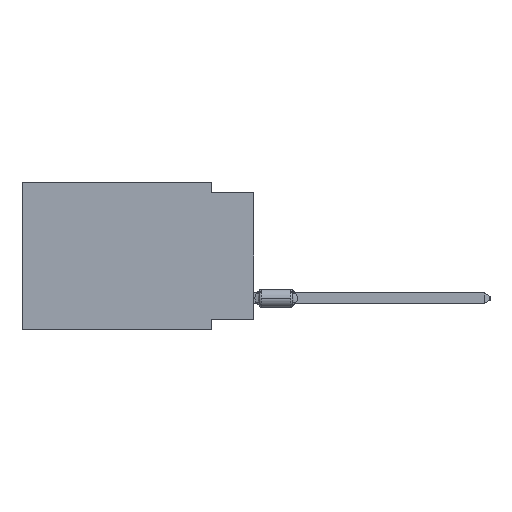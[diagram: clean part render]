
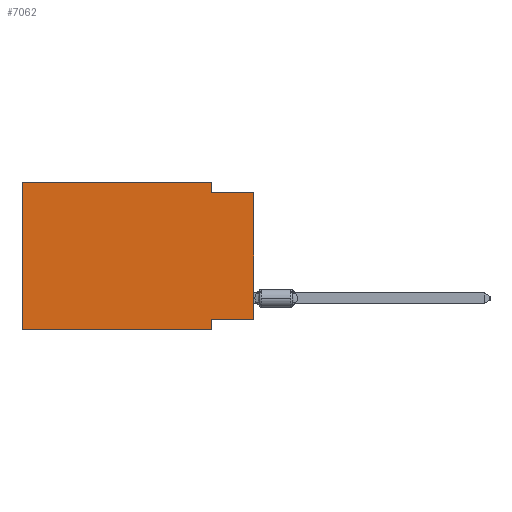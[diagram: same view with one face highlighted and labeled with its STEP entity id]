
A CAD part, left-side view. The second image highlights one B-rep face of the part: STEP entity #7062.
In plain terms, the highlighted planar face has unit normal (-1, 0, 0).
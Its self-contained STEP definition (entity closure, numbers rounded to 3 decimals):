
#472 = EDGE_CURVE ( 'NONE', #13947, #16221, #6965, .T. ) ;
#682 = CARTESIAN_POINT ( 'NONE',  ( 0., 2.54, -0.635 ) ) ;
#1280 = CARTESIAN_POINT ( 'NONE',  ( 0., 0., -8.255 ) ) ;
#1526 = VECTOR ( 'NONE', #20404, 1000. ) ;
#2640 = EDGE_CURVE ( 'NONE', #15293, #5087, #4726, .T. ) ;
#2750 = EDGE_CURVE ( 'NONE', #7105, #22051, #5761, .T. ) ;
#4482 = VECTOR ( 'NONE', #26361, 1000. ) ;
#4726 = LINE ( 'NONE', #29199, #33858 ) ;
#5087 = VERTEX_POINT ( 'NONE', #25525 ) ;
#5761 = LINE ( 'NONE', #30059, #32177 ) ;
#6753 = LINE ( 'NONE', #9949, #7894 ) ;
#6858 = CARTESIAN_POINT ( 'NONE',  ( 0., 2.54, -8.89 ) ) ;
#6965 = LINE ( 'NONE', #9617, #29930 ) ;
#7062 = ADVANCED_FACE ( 'NONE', ( #32256 ), #7942, .F. ) ;
#7105 = VERTEX_POINT ( 'NONE', #22108 ) ;
#7195 = CARTESIAN_POINT ( 'NONE',  ( 0., 2.54, -8.255 ) ) ;
#7276 = DIRECTION ( 'NONE',  ( 0., 0., 1. ) ) ;
#7894 = VECTOR ( 'NONE', #7276, 1000. ) ;
#7942 = PLANE ( 'NONE',  #29981 ) ;
#8494 = EDGE_CURVE ( 'NONE', #22051, #16221, #18554, .T. ) ;
#9617 = CARTESIAN_POINT ( 'NONE',  ( 0., 0., 0. ) ) ;
#9874 = CARTESIAN_POINT ( 'NONE',  ( 0., 0., -0.635 ) ) ;
#9949 = CARTESIAN_POINT ( 'NONE',  ( 0., 13.97, 0. ) ) ;
#10216 = DIRECTION ( 'NONE',  ( 0., -1., 0. ) ) ;
#10728 = LINE ( 'NONE', #18544, #23332 ) ;
#12351 = DIRECTION ( 'NONE',  ( 0., 0., -1. ) ) ;
#12428 = LINE ( 'NONE', #26437, #1526 ) ;
#12834 = ORIENTED_EDGE ( 'NONE', *, *, #33406, .F. ) ;
#13947 = VERTEX_POINT ( 'NONE', #1280 ) ;
#15293 = VERTEX_POINT ( 'NONE', #19280 ) ;
#15492 = VECTOR ( 'NONE', #12351, 1000. ) ;
#15493 = DIRECTION ( 'NONE',  ( 0., 0., 1. ) ) ;
#16221 = VERTEX_POINT ( 'NONE', #20080 ) ;
#16418 = ORIENTED_EDGE ( 'NONE', *, *, #18276, .F. ) ;
#17392 = VERTEX_POINT ( 'NONE', #7195 ) ;
#18276 = EDGE_CURVE ( 'NONE', #13947, #17392, #12428, .T. ) ;
#18544 = CARTESIAN_POINT ( 'NONE',  ( 0., 13.97, 0. ) ) ;
#18554 = LINE ( 'NONE', #9874, #4482 ) ;
#18767 = CARTESIAN_POINT ( 'NONE',  ( 0., 13.97, 0. ) ) ;
#19280 = CARTESIAN_POINT ( 'NONE',  ( 0., 13.97, -8.89 ) ) ;
#20080 = CARTESIAN_POINT ( 'NONE',  ( 0., 0., -0.635 ) ) ;
#20404 = DIRECTION ( 'NONE',  ( 0., 1., 0. ) ) ;
#22051 = VERTEX_POINT ( 'NONE', #682 ) ;
#22108 = CARTESIAN_POINT ( 'NONE',  ( 0., 2.54, 0. ) ) ;
#22488 = ORIENTED_EDGE ( 'NONE', *, *, #8494, .F. ) ;
#23332 = VECTOR ( 'NONE', #34875, 1000. ) ;
#23356 = EDGE_LOOP ( 'NONE', ( #32543, #22488, #24881, #31233, #24174, #25455, #12834, #16418 ) ) ;
#24174 = ORIENTED_EDGE ( 'NONE', *, *, #27431, .F. ) ;
#24247 = DIRECTION ( 'NONE',  ( 1., 0., 0. ) ) ;
#24881 = ORIENTED_EDGE ( 'NONE', *, *, #2750, .F. ) ;
#25455 = ORIENTED_EDGE ( 'NONE', *, *, #2640, .T. ) ;
#25525 = CARTESIAN_POINT ( 'NONE',  ( 0., 2.54, -8.89 ) ) ;
#26361 = DIRECTION ( 'NONE',  ( 0., -1., 0. ) ) ;
#26437 = CARTESIAN_POINT ( 'NONE',  ( 0., 0., -8.255 ) ) ;
#27431 = EDGE_CURVE ( 'NONE', #15293, #32837, #6753, .T. ) ;
#27482 = CARTESIAN_POINT ( 'NONE',  ( 0., 13.97, 0. ) ) ;
#29199 = CARTESIAN_POINT ( 'NONE',  ( 0., 13.97, -8.89 ) ) ;
#29930 = VECTOR ( 'NONE', #15493, 1000. ) ;
#29981 = AXIS2_PLACEMENT_3D ( 'NONE', #18767, #24247, #35083 ) ;
#30059 = CARTESIAN_POINT ( 'NONE',  ( 0., 2.54, 0. ) ) ;
#30709 = EDGE_CURVE ( 'NONE', #32837, #7105, #10728, .T. ) ;
#31233 = ORIENTED_EDGE ( 'NONE', *, *, #30709, .F. ) ;
#31346 = LINE ( 'NONE', #6858, #15492 ) ;
#32177 = VECTOR ( 'NONE', #34883, 1000. ) ;
#32256 = FACE_OUTER_BOUND ( 'NONE', #23356, .T. ) ;
#32543 = ORIENTED_EDGE ( 'NONE', *, *, #472, .T. ) ;
#32837 = VERTEX_POINT ( 'NONE', #27482 ) ;
#33406 = EDGE_CURVE ( 'NONE', #17392, #5087, #31346, .T. ) ;
#33858 = VECTOR ( 'NONE', #10216, 1000. ) ;
#34875 = DIRECTION ( 'NONE',  ( 0., -1., 0. ) ) ;
#34883 = DIRECTION ( 'NONE',  ( 0., 0., -1. ) ) ;
#35083 = DIRECTION ( 'NONE',  ( 0., 0., -1. ) ) ;
